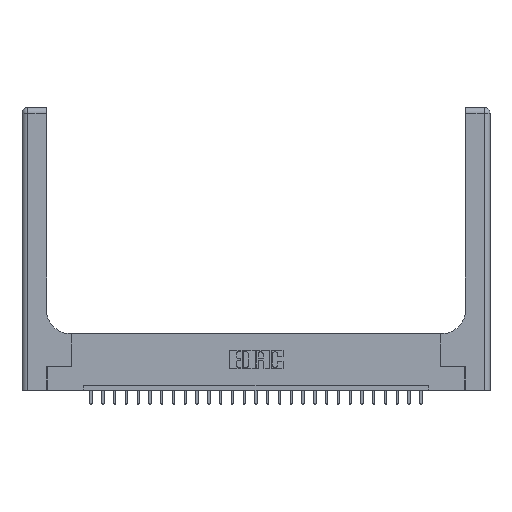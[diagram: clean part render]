
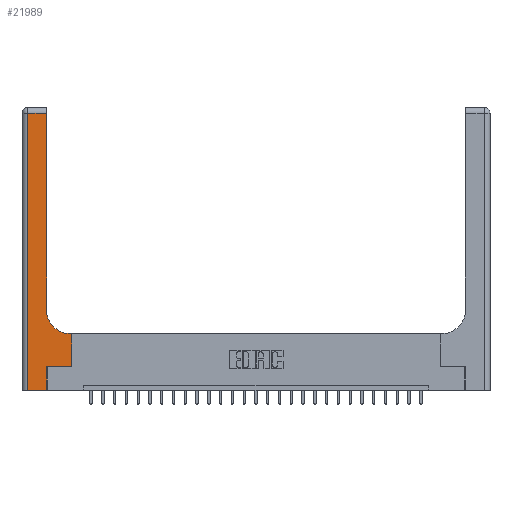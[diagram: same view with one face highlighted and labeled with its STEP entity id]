
A CAD part, top view. The second image highlights one B-rep face of the part: STEP entity #21989.
In plain terms, the highlighted planar face has unit normal (0, 0, 1).
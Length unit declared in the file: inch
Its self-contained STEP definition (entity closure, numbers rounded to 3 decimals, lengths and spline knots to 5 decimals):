
#383 = CARTESIAN_POINT ( 'NONE',  ( 0.265, 0., 0.37 ) ) ;
#494 = VECTOR ( 'NONE', #1531, 39.37008 ) ;
#561 = EDGE_CURVE ( 'NONE', #14725, #17049, #20882, .T. ) ;
#853 = CARTESIAN_POINT ( 'NONE',  ( 0.26, 2.94, 0.37 ) ) ;
#1429 = FACE_OUTER_BOUND ( 'NONE', #25392, .T. ) ;
#1531 = DIRECTION ( 'NONE',  ( -1., 0., 0. ) ) ;
#1972 = ORIENTED_EDGE ( 'NONE', *, *, #24604, .T. ) ;
#2044 = VECTOR ( 'NONE', #7775, 39.37008 ) ;
#2213 = CARTESIAN_POINT ( 'NONE',  ( 0., 0., 0.37 ) ) ;
#2464 = DIRECTION ( 'NONE',  ( 1., 0., 0. ) ) ;
#3353 = DIRECTION ( 'NONE',  ( 0., 0., -1. ) ) ;
#4220 = VERTEX_POINT ( 'NONE', #4931 ) ;
#4367 = DIRECTION ( 'NONE',  ( 0., 1., 0. ) ) ;
#4931 = CARTESIAN_POINT ( 'NONE',  ( 0.26, 0.85, 0.37 ) ) ;
#5024 = AXIS2_PLACEMENT_3D ( 'NONE', #9912, #21844, #23768 ) ;
#5303 = EDGE_CURVE ( 'NONE', #16317, #15983, #21892, .T. ) ;
#5399 = CARTESIAN_POINT ( 'NONE',  ( 0.26, 0.6, 0.37 ) ) ;
#5528 = LINE ( 'NONE', #5399, #494 ) ;
#5555 = ORIENTED_EDGE ( 'NONE', *, *, #561, .T. ) ;
#6331 = CARTESIAN_POINT ( 'NONE',  ( 0.26, 3., 0.37 ) ) ;
#7029 = CARTESIAN_POINT ( 'NONE',  ( 0.265, 0.25, 0.37 ) ) ;
#7553 = ORIENTED_EDGE ( 'NONE', *, *, #17820, .T. ) ;
#7602 = LINE ( 'NONE', #11571, #22873 ) ;
#7775 = DIRECTION ( 'NONE',  ( 0., -1., 0. ) ) ;
#9272 = PLANE ( 'NONE',  #22620 ) ;
#9912 = CARTESIAN_POINT ( 'NONE',  ( 0.51, 0.85, 0.37 ) ) ;
#10523 = VECTOR ( 'NONE', #18569, 39.37008 ) ;
#10683 = VECTOR ( 'NONE', #17670, 39.37008 ) ;
#10827 = VERTEX_POINT ( 'NONE', #853 ) ;
#11525 = EDGE_CURVE ( 'NONE', #4220, #10827, #21988, .T. ) ;
#11571 = CARTESIAN_POINT ( 'NONE',  ( 0., 2.94, 0.37 ) ) ;
#11646 = CARTESIAN_POINT ( 'NONE',  ( 0.528, 0.25, 0.37 ) ) ;
#12462 = ORIENTED_EDGE ( 'NONE', *, *, #12887, .T. ) ;
#12887 = EDGE_CURVE ( 'NONE', #15983, #13679, #15828, .T. ) ;
#13539 = ORIENTED_EDGE ( 'NONE', *, *, #17695, .T. ) ;
#13548 = CARTESIAN_POINT ( 'NONE',  ( 0.06, 3., 0.37 ) ) ;
#13664 = VERTEX_POINT ( 'NONE', #25290 ) ;
#13679 = VERTEX_POINT ( 'NONE', #21182 ) ;
#13948 = LINE ( 'NONE', #11646, #10683 ) ;
#14725 = VERTEX_POINT ( 'NONE', #23499 ) ;
#14912 = CARTESIAN_POINT ( 'NONE',  ( 0.51, 0.6, 0.37 ) ) ;
#15083 = VECTOR ( 'NONE', #4367, 39.37008 ) ;
#15453 = ORIENTED_EDGE ( 'NONE', *, *, #11525, .T. ) ;
#15828 = LINE ( 'NONE', #2213, #21116 ) ;
#15903 = ORIENTED_EDGE ( 'NONE', *, *, #21155, .T. ) ;
#15983 = VERTEX_POINT ( 'NONE', #17241 ) ;
#16317 = VERTEX_POINT ( 'NONE', #16669 ) ;
#16669 = CARTESIAN_POINT ( 'NONE',  ( 0.06, 2.94, 0.37 ) ) ;
#16775 = LINE ( 'NONE', #383, #15083 ) ;
#17049 = VERTEX_POINT ( 'NONE', #18400 ) ;
#17241 = CARTESIAN_POINT ( 'NONE',  ( 0.06, 0., 0.37 ) ) ;
#17670 = DIRECTION ( 'NONE',  ( 0., 1., 0. ) ) ;
#17695 = EDGE_CURVE ( 'NONE', #10827, #16317, #7602, .T. ) ;
#17729 = CIRCLE ( 'NONE', #5024, 0.25 ) ;
#17820 = EDGE_CURVE ( 'NONE', #13679, #14725, #16775, .T. ) ;
#18400 = CARTESIAN_POINT ( 'NONE',  ( 0.528, 0.25, 0.37 ) ) ;
#18569 = DIRECTION ( 'NONE',  ( 1., 0., 0. ) ) ;
#18725 = ORIENTED_EDGE ( 'NONE', *, *, #24899, .T. ) ;
#19401 = DIRECTION ( 'NONE',  ( -1., 0., 0. ) ) ;
#20055 = DIRECTION ( 'NONE',  ( 0., 1., 0. ) ) ;
#20574 = CARTESIAN_POINT ( 'NONE',  ( 0., 3., 0.37 ) ) ;
#20882 = LINE ( 'NONE', #7029, #10523 ) ;
#21078 = DIRECTION ( 'NONE',  ( -1., 0., 0. ) ) ;
#21116 = VECTOR ( 'NONE', #2464, 39.37008 ) ;
#21155 = EDGE_CURVE ( 'NONE', #17049, #13664, #13948, .T. ) ;
#21182 = CARTESIAN_POINT ( 'NONE',  ( 0.265, 0., 0.37 ) ) ;
#21844 = DIRECTION ( 'NONE',  ( 0., 0., -1. ) ) ;
#21892 = LINE ( 'NONE', #13548, #2044 ) ;
#21988 = LINE ( 'NONE', #6331, #23541 ) ;
#21989 = ADVANCED_FACE ( 'NONE', ( #1429 ), #9272, .F. ) ;
#22620 = AXIS2_PLACEMENT_3D ( 'NONE', #20574, #3353, #21078 ) ;
#22873 = VECTOR ( 'NONE', #19401, 39.37008 ) ;
#23499 = CARTESIAN_POINT ( 'NONE',  ( 0.265, 0.25, 0.37 ) ) ;
#23541 = VECTOR ( 'NONE', #20055, 39.37008 ) ;
#23768 = DIRECTION ( 'NONE',  ( 1., 0., 0. ) ) ;
#24604 = EDGE_CURVE ( 'NONE', #25364, #4220, #17729, .T. ) ;
#24899 = EDGE_CURVE ( 'NONE', #13664, #25364, #5528, .T. ) ;
#25244 = ORIENTED_EDGE ( 'NONE', *, *, #5303, .T. ) ;
#25290 = CARTESIAN_POINT ( 'NONE',  ( 0.528, 0.6, 0.37 ) ) ;
#25364 = VERTEX_POINT ( 'NONE', #14912 ) ;
#25392 = EDGE_LOOP ( 'NONE', ( #15453, #13539, #25244, #12462, #7553, #5555, #15903, #18725, #1972 ) ) ;
